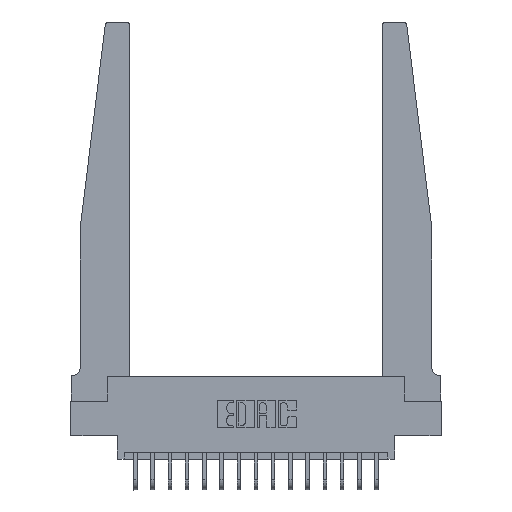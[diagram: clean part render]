
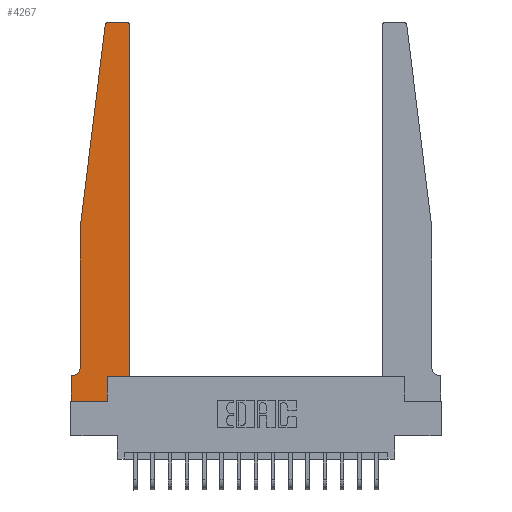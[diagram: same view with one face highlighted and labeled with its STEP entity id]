
A CAD part, top view. The second image highlights one B-rep face of the part: STEP entity #4267.
In plain terms, the highlighted planar face has unit normal (0, 0, 1).
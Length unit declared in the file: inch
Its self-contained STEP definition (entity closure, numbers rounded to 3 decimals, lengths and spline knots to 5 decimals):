
#422 = DIRECTION ( 'NONE',  ( 0., -1., 0. ) ) ;
#453 = LINE ( 'NONE', #7831, #4600 ) ;
#736 = DIRECTION ( 'NONE',  ( -1., 0., 0. ) ) ;
#903 = CARTESIAN_POINT ( 'NONE',  ( 0.425, 0.18, 0.37 ) ) ;
#1520 = CARTESIAN_POINT ( 'NONE',  ( 0.395, 2.72, 0.37 ) ) ;
#1563 = ORIENTED_EDGE ( 'NONE', *, *, #18234, .T. ) ;
#1603 = DIRECTION ( 'NONE',  ( 0., 0., 1. ) ) ;
#1779 = ORIENTED_EDGE ( 'NONE', *, *, #11915, .T. ) ;
#1878 = CARTESIAN_POINT ( 'NONE',  ( 0.395, 2.75, 0.37 ) ) ;
#1961 = CARTESIAN_POINT ( 'NONE',  ( 0.27653, 2.72, 0.37 ) ) ;
#2134 = CARTESIAN_POINT ( 'NONE',  ( 0.2605, 0., 0.37 ) ) ;
#2243 = EDGE_CURVE ( 'NONE', #14964, #4972, #9254, .T. ) ;
#2410 = EDGE_CURVE ( 'NONE', #9376, #3949, #6109, .T. ) ;
#2796 = VERTEX_POINT ( 'NONE', #14734 ) ;
#3014 = DIRECTION ( 'NONE',  ( 1., 0., 0. ) ) ;
#3032 = VERTEX_POINT ( 'NONE', #11021 ) ;
#3125 = CARTESIAN_POINT ( 'NONE',  ( 0.065, 1.25, 0.37 ) ) ;
#3518 = DIRECTION ( 'NONE',  ( 0., -1., 0. ) ) ;
#3949 = VERTEX_POINT ( 'NONE', #17494 ) ;
#4103 = LINE ( 'NONE', #7927, #12128 ) ;
#4267 = ADVANCED_FACE ( 'NONE', ( #15122 ), #6020, .T. ) ;
#4482 = LINE ( 'NONE', #18822, #9479 ) ;
#4589 = ORIENTED_EDGE ( 'NONE', *, *, #2410, .T. ) ;
#4600 = VECTOR ( 'NONE', #6578, 39.37008 ) ;
#4627 = CIRCLE ( 'NONE', #10048, 0.03 ) ;
#4657 = VECTOR ( 'NONE', #7441, 39.37008 ) ;
#4659 = VERTEX_POINT ( 'NONE', #18249 ) ;
#4972 = VERTEX_POINT ( 'NONE', #19661 ) ;
#5316 = DIRECTION ( 'NONE',  ( 0., 0., -1. ) ) ;
#5608 = LINE ( 'NONE', #17739, #12427 ) ;
#5637 = ORIENTED_EDGE ( 'NONE', *, *, #2243, .T. ) ;
#5999 = EDGE_CURVE ( 'NONE', #3949, #12135, #453, .T. ) ;
#6020 = PLANE ( 'NONE',  #6434 ) ;
#6079 = ORIENTED_EDGE ( 'NONE', *, *, #12581, .T. ) ;
#6109 = CIRCLE ( 'NONE', #9768, 0.05 ) ;
#6203 = VERTEX_POINT ( 'NONE', #7880 ) ;
#6434 = AXIS2_PLACEMENT_3D ( 'NONE', #18649, #1603, #18581 ) ;
#6578 = DIRECTION ( 'NONE',  ( -1., 0., 0. ) ) ;
#6590 = DIRECTION ( 'NONE',  ( 0., 0., 1. ) ) ;
#6830 = VECTOR ( 'NONE', #7913, 39.37008 ) ;
#6928 = EDGE_CURVE ( 'NONE', #12135, #3032, #4103, .T. ) ;
#7405 = ORIENTED_EDGE ( 'NONE', *, *, #13283, .T. ) ;
#7428 = CARTESIAN_POINT ( 'NONE',  ( 0.425, 0.18, 0.37 ) ) ;
#7441 = DIRECTION ( 'NONE',  ( 1., 0., 0. ) ) ;
#7650 = CARTESIAN_POINT ( 'NONE',  ( 0., 0.1875, 0.37 ) ) ;
#7831 = CARTESIAN_POINT ( 'NONE',  ( 0.065, 0.1875, 0.37 ) ) ;
#7880 = CARTESIAN_POINT ( 'NONE',  ( 0.24675, 2.72367, 0.37 ) ) ;
#7913 = DIRECTION ( 'NONE',  ( -1., 0., 0. ) ) ;
#7927 = CARTESIAN_POINT ( 'NONE',  ( 0., 0., 0.37 ) ) ;
#8144 = ORIENTED_EDGE ( 'NONE', *, *, #6928, .T. ) ;
#8597 = DIRECTION ( 'NONE',  ( 1., 0., 0. ) ) ;
#8676 = CARTESIAN_POINT ( 'NONE',  ( 0.425, 0.18, 0.37 ) ) ;
#8680 = EDGE_CURVE ( 'NONE', #4659, #9376, #9138, .T. ) ;
#8701 = LINE ( 'NONE', #8676, #17514 ) ;
#8869 = ORIENTED_EDGE ( 'NONE', *, *, #8680, .T. ) ;
#8887 = VECTOR ( 'NONE', #3518, 39.37008 ) ;
#9138 = LINE ( 'NONE', #3125, #8887 ) ;
#9254 = LINE ( 'NONE', #12489, #6830 ) ;
#9376 = VERTEX_POINT ( 'NONE', #13202 ) ;
#9479 = VECTOR ( 'NONE', #18755, 39.37008 ) ;
#9701 = VERTEX_POINT ( 'NONE', #2134 ) ;
#9768 = AXIS2_PLACEMENT_3D ( 'NONE', #11597, #5316, #736 ) ;
#9800 = EDGE_LOOP ( 'NONE', ( #5637, #1563, #6079, #8869, #4589, #15427, #8144, #1779, #18459, #20047, #7405, #19003 ) ) ;
#9970 = CIRCLE ( 'NONE', #16623, 0.03 ) ;
#9983 = LINE ( 'NONE', #11674, #14823 ) ;
#10048 = AXIS2_PLACEMENT_3D ( 'NONE', #1961, #6590, #11476 ) ;
#10697 = EDGE_CURVE ( 'NONE', #9701, #14068, #4482, .T. ) ;
#11021 = CARTESIAN_POINT ( 'NONE',  ( 0., 0., 0.37 ) ) ;
#11118 = EDGE_CURVE ( 'NONE', #14068, #11649, #16592, .T. ) ;
#11476 = DIRECTION ( 'NONE',  ( 1., 0., 0. ) ) ;
#11597 = CARTESIAN_POINT ( 'NONE',  ( 0.015, 0.2375, 0.37 ) ) ;
#11649 = VERTEX_POINT ( 'NONE', #7428 ) ;
#11674 = CARTESIAN_POINT ( 'NONE',  ( 0.065, 1.25, 0.37 ) ) ;
#11915 = EDGE_CURVE ( 'NONE', #3032, #9701, #5608, .T. ) ;
#12128 = VECTOR ( 'NONE', #422, 39.37008 ) ;
#12135 = VERTEX_POINT ( 'NONE', #7650 ) ;
#12396 = DIRECTION ( 'NONE',  ( 0., 0., 1. ) ) ;
#12427 = VECTOR ( 'NONE', #8597, 39.37008 ) ;
#12489 = CARTESIAN_POINT ( 'NONE',  ( 0.25, 2.75, 0.37 ) ) ;
#12581 = EDGE_CURVE ( 'NONE', #6203, #4659, #9983, .T. ) ;
#12874 = EDGE_CURVE ( 'NONE', #2796, #14964, #9970, .T. ) ;
#13202 = CARTESIAN_POINT ( 'NONE',  ( 0.065, 0.2375, 0.37 ) ) ;
#13283 = EDGE_CURVE ( 'NONE', #11649, #2796, #8701, .T. ) ;
#14068 = VERTEX_POINT ( 'NONE', #16232 ) ;
#14734 = CARTESIAN_POINT ( 'NONE',  ( 0.425, 2.72, 0.37 ) ) ;
#14823 = VECTOR ( 'NONE', #19571, 39.37008 ) ;
#14964 = VERTEX_POINT ( 'NONE', #1878 ) ;
#15122 = FACE_OUTER_BOUND ( 'NONE', #9800, .T. ) ;
#15427 = ORIENTED_EDGE ( 'NONE', *, *, #5999, .T. ) ;
#16232 = CARTESIAN_POINT ( 'NONE',  ( 0.2605, 0.18, 0.37 ) ) ;
#16592 = LINE ( 'NONE', #903, #4657 ) ;
#16623 = AXIS2_PLACEMENT_3D ( 'NONE', #1520, #12396, #3014 ) ;
#17494 = CARTESIAN_POINT ( 'NONE',  ( 0.015, 0.1875, 0.37 ) ) ;
#17514 = VECTOR ( 'NONE', #19675, 39.37008 ) ;
#17739 = CARTESIAN_POINT ( 'NONE',  ( 0., 0., 0.37 ) ) ;
#18234 = EDGE_CURVE ( 'NONE', #4972, #6203, #4627, .T. ) ;
#18249 = CARTESIAN_POINT ( 'NONE',  ( 0.065, 1.25, 0.37 ) ) ;
#18459 = ORIENTED_EDGE ( 'NONE', *, *, #10697, .T. ) ;
#18581 = DIRECTION ( 'NONE',  ( 1., 0., 0. ) ) ;
#18649 = CARTESIAN_POINT ( 'NONE',  ( 0., 0.1875, 0.37 ) ) ;
#18755 = DIRECTION ( 'NONE',  ( 0., 1., 0. ) ) ;
#18822 = CARTESIAN_POINT ( 'NONE',  ( 0.2605, 0.18, 0.37 ) ) ;
#19003 = ORIENTED_EDGE ( 'NONE', *, *, #12874, .T. ) ;
#19571 = DIRECTION ( 'NONE',  ( -0.122, -0.992, 0. ) ) ;
#19661 = CARTESIAN_POINT ( 'NONE',  ( 0.27653, 2.75, 0.37 ) ) ;
#19675 = DIRECTION ( 'NONE',  ( 0., 1., 0. ) ) ;
#20047 = ORIENTED_EDGE ( 'NONE', *, *, #11118, .T. ) ;
